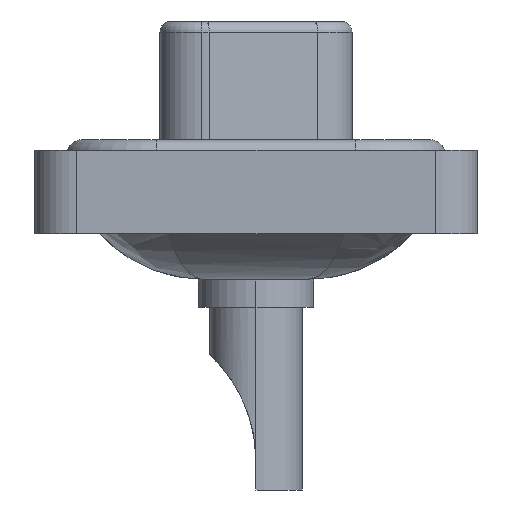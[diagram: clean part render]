
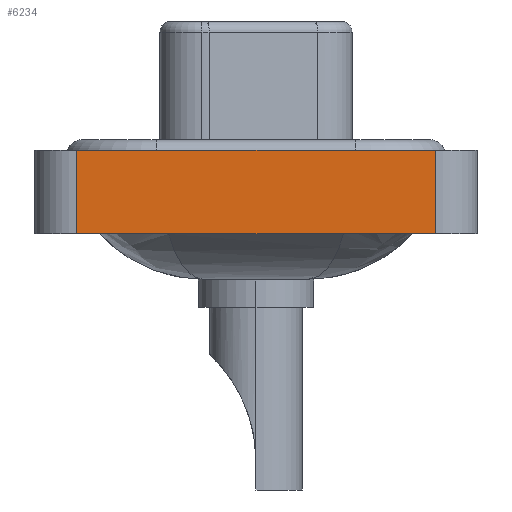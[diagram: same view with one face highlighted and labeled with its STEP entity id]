
A CAD part, left-side view. The second image highlights one B-rep face of the part: STEP entity #6234.
In plain terms, the highlighted planar face has unit normal (-1, 0, 0).
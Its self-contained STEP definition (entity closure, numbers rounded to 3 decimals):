
#673 = CARTESIAN_POINT ( 'NONE',  ( -7.35, -8.55, -3.6 ) ) ;
#963 = FACE_OUTER_BOUND ( 'NONE', #16072, .T. ) ;
#1149 = CARTESIAN_POINT ( 'NONE',  ( -7.35, 8.55, -3.6 ) ) ;
#2224 = EDGE_CURVE ( 'NONE', #15687, #18789, #22400, .T. ) ;
#2602 = EDGE_CURVE ( 'NONE', #18562, #15687, #9192, .T. ) ;
#4265 = CARTESIAN_POINT ( 'NONE',  ( -7.35, -8.55, -3.6 ) ) ;
#5408 = DIRECTION ( 'NONE',  ( 0., -1., 0. ) ) ;
#6234 = ADVANCED_FACE ( 'NONE', ( #963 ), #16297, .T. ) ;
#6688 = CARTESIAN_POINT ( 'NONE',  ( -7.35, -8.55, -3.6 ) ) ;
#7345 = VECTOR ( 'NONE', #9522, 1000. ) ;
#7538 = ORIENTED_EDGE ( 'NONE', *, *, #2602, .T. ) ;
#7672 = DIRECTION ( 'NONE',  ( 0., 0., 1. ) ) ;
#8079 = VECTOR ( 'NONE', #18327, 1000. ) ;
#8815 = LINE ( 'NONE', #20981, #19052 ) ;
#9192 = LINE ( 'NONE', #673, #7345 ) ;
#9522 = DIRECTION ( 'NONE',  ( 0., -1., 0. ) ) ;
#10047 = ORIENTED_EDGE ( 'NONE', *, *, #2224, .T. ) ;
#10352 = CARTESIAN_POINT ( 'NONE',  ( -7.35, 8.55, -3.6 ) ) ;
#10359 = ORIENTED_EDGE ( 'NONE', *, *, #13320, .F. ) ;
#11687 = CARTESIAN_POINT ( 'NONE',  ( -7.35, -8.55, -3.6 ) ) ;
#12034 = VERTEX_POINT ( 'NONE', #21349 ) ;
#12781 = VECTOR ( 'NONE', #22174, 1000. ) ;
#13320 = EDGE_CURVE ( 'NONE', #12034, #18789, #8815, .T. ) ;
#15071 = EDGE_CURVE ( 'NONE', #18562, #12034, #21751, .T. ) ;
#15687 = VERTEX_POINT ( 'NONE', #6688 ) ;
#16072 = EDGE_LOOP ( 'NONE', ( #10047, #10359, #17350, #7538 ) ) ;
#16297 = PLANE ( 'NONE',  #16902 ) ;
#16512 = DIRECTION ( 'NONE',  ( -1., 0., 0. ) ) ;
#16902 = AXIS2_PLACEMENT_3D ( 'NONE', #4265, #16512, #7672 ) ;
#17350 = ORIENTED_EDGE ( 'NONE', *, *, #15071, .F. ) ;
#18327 = DIRECTION ( 'NONE',  ( 0., 0., 1. ) ) ;
#18435 = CARTESIAN_POINT ( 'NONE',  ( -7.35, -8.55, 0.4 ) ) ;
#18562 = VERTEX_POINT ( 'NONE', #10352 ) ;
#18789 = VERTEX_POINT ( 'NONE', #18435 ) ;
#19052 = VECTOR ( 'NONE', #5408, 1000. ) ;
#20981 = CARTESIAN_POINT ( 'NONE',  ( -7.35, -8.55, 0.4 ) ) ;
#21349 = CARTESIAN_POINT ( 'NONE',  ( -7.35, 8.55, 0.4 ) ) ;
#21751 = LINE ( 'NONE', #1149, #8079 ) ;
#22174 = DIRECTION ( 'NONE',  ( 0., 0., 1. ) ) ;
#22400 = LINE ( 'NONE', #11687, #12781 ) ;
